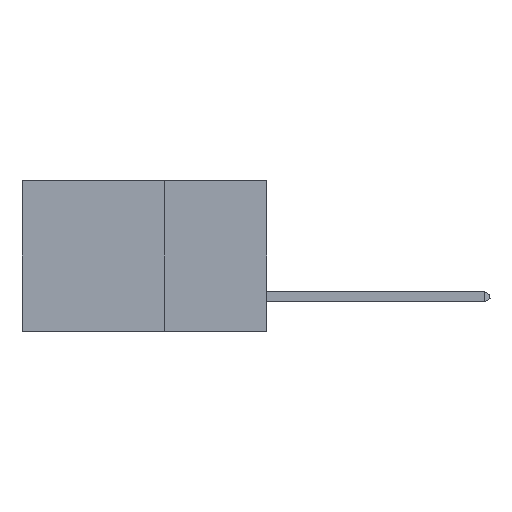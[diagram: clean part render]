
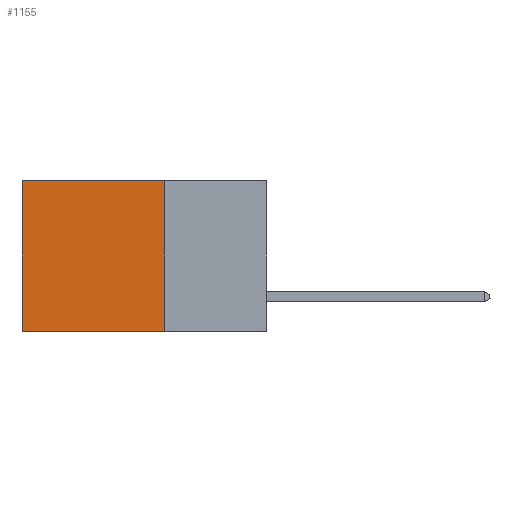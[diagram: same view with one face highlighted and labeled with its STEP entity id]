
A CAD part, left-side view. The second image highlights one B-rep face of the part: STEP entity #1155.
In plain terms, the highlighted planar face has unit normal (-1, 0, 0).
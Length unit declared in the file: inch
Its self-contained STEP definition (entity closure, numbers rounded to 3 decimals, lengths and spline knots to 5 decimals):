
#67 = EDGE_LOOP ( 'NONE', ( #2705, #4129, #842, #5995 ) ) ;
#398 = CARTESIAN_POINT ( 'NONE',  ( 0.2875, 0.25, 0. ) ) ;
#792 = CARTESIAN_POINT ( 'NONE',  ( 0.2875, 0.6, 0. ) ) ;
#842 = ORIENTED_EDGE ( 'NONE', *, *, #10553, .F. ) ;
#849 = AXIS2_PLACEMENT_3D ( 'NONE', #10994, #8760, #7823 ) ;
#1155 = ADVANCED_FACE ( 'NONE', ( #10018 ), #5011, .F. ) ;
#1655 = LINE ( 'NONE', #4742, #5123 ) ;
#2705 = ORIENTED_EDGE ( 'NONE', *, *, #5815, .T. ) ;
#3111 = EDGE_CURVE ( 'NONE', #11193, #3305, #4296, .T. ) ;
#3137 = VERTEX_POINT ( 'NONE', #8214 ) ;
#3305 = VERTEX_POINT ( 'NONE', #6911 ) ;
#3450 = DIRECTION ( 'NONE',  ( 0., 1., 0. ) ) ;
#3860 = CARTESIAN_POINT ( 'NONE',  ( 0.2875, 0.25, 0. ) ) ;
#4129 = ORIENTED_EDGE ( 'NONE', *, *, #8546, .F. ) ;
#4296 = LINE ( 'NONE', #398, #9241 ) ;
#4335 = LINE ( 'NONE', #7963, #6378 ) ;
#4742 = CARTESIAN_POINT ( 'NONE',  ( 0.2875, 0.25, -0.37 ) ) ;
#5011 = PLANE ( 'NONE',  #849 ) ;
#5123 = VECTOR ( 'NONE', #6688, 39.37008 ) ;
#5815 = EDGE_CURVE ( 'NONE', #3305, #3137, #5980, .T. ) ;
#5980 = LINE ( 'NONE', #792, #6420 ) ;
#5995 = ORIENTED_EDGE ( 'NONE', *, *, #3111, .T. ) ;
#6378 = VECTOR ( 'NONE', #9846, 39.37008 ) ;
#6420 = VECTOR ( 'NONE', #9331, 39.37008 ) ;
#6501 = VERTEX_POINT ( 'NONE', #7604 ) ;
#6688 = DIRECTION ( 'NONE',  ( 0., 1., 0. ) ) ;
#6911 = CARTESIAN_POINT ( 'NONE',  ( 0.2875, 0.6, 0. ) ) ;
#7604 = CARTESIAN_POINT ( 'NONE',  ( 0.2875, 0.25, -0.37 ) ) ;
#7823 = DIRECTION ( 'NONE',  ( 0., 0., -1. ) ) ;
#7963 = CARTESIAN_POINT ( 'NONE',  ( 0.2875, 0.25, 0. ) ) ;
#8214 = CARTESIAN_POINT ( 'NONE',  ( 0.2875, 0.6, -0.37 ) ) ;
#8546 = EDGE_CURVE ( 'NONE', #6501, #3137, #1655, .T. ) ;
#8760 = DIRECTION ( 'NONE',  ( 1., 0., 0. ) ) ;
#9241 = VECTOR ( 'NONE', #3450, 39.37008 ) ;
#9331 = DIRECTION ( 'NONE',  ( 0., 0., -1. ) ) ;
#9846 = DIRECTION ( 'NONE',  ( 0., 0., -1. ) ) ;
#10018 = FACE_OUTER_BOUND ( 'NONE', #67, .T. ) ;
#10553 = EDGE_CURVE ( 'NONE', #11193, #6501, #4335, .T. ) ;
#10994 = CARTESIAN_POINT ( 'NONE',  ( 0.2875, 0.25, 0. ) ) ;
#11193 = VERTEX_POINT ( 'NONE', #3860 ) ;
